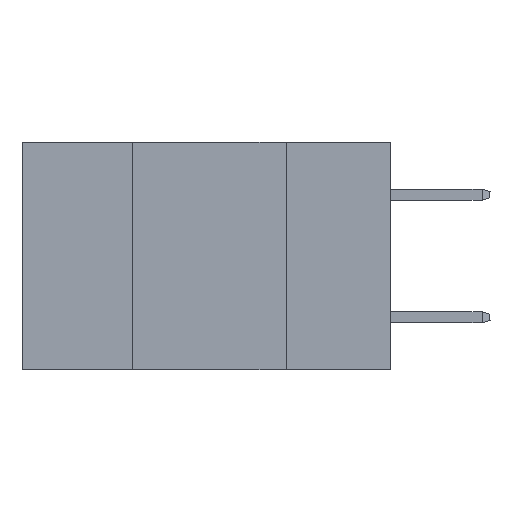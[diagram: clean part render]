
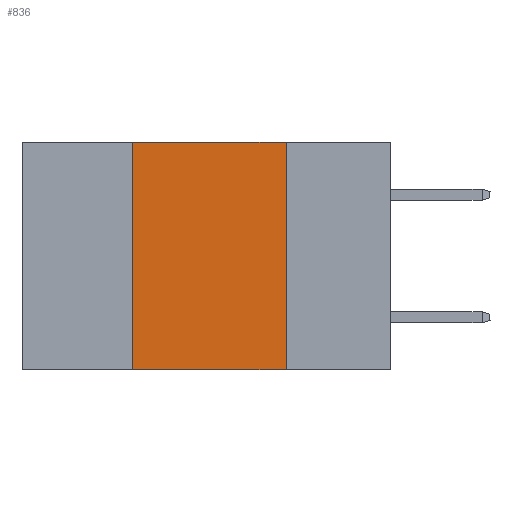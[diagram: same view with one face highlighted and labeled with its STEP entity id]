
A CAD part, left-side view. The second image highlights one B-rep face of the part: STEP entity #836.
In plain terms, the highlighted planar face has unit normal (-1, 0, 0).
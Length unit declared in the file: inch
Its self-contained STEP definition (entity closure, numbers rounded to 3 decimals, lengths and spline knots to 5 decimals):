
#183 = ORIENTED_EDGE ( 'NONE', *, *, #1083, .F. ) ;
#836 = ADVANCED_FACE ( 'NONE', ( #3090 ), #2883, .F. ) ;
#1083 = EDGE_CURVE ( 'NONE', #12648, #2559, #15707, .T. ) ;
#1104 = CARTESIAN_POINT ( 'NONE',  ( 0., 0.42, -0.37 ) ) ;
#1356 = DIRECTION ( 'NONE',  ( 0., -1., 0. ) ) ;
#1538 = EDGE_CURVE ( 'NONE', #8783, #17082, #5696, .T. ) ;
#1932 = VECTOR ( 'NONE', #1356, 39.37008 ) ;
#2559 = VERTEX_POINT ( 'NONE', #19711 ) ;
#2883 = PLANE ( 'NONE',  #14204 ) ;
#3090 = FACE_OUTER_BOUND ( 'NONE', #19800, .T. ) ;
#3466 = CARTESIAN_POINT ( 'NONE',  ( 0., 0.42, 0. ) ) ;
#3748 = EDGE_CURVE ( 'NONE', #12648, #17082, #10175, .T. ) ;
#4660 = CARTESIAN_POINT ( 'NONE',  ( 0., 0.17, -0.37 ) ) ;
#4738 = DIRECTION ( 'NONE',  ( 0., 0., -1. ) ) ;
#5691 = DIRECTION ( 'NONE',  ( 0., -1., 0. ) ) ;
#5696 = LINE ( 'NONE', #6058, #16393 ) ;
#5962 = VECTOR ( 'NONE', #6739, 39.37008 ) ;
#6058 = CARTESIAN_POINT ( 'NONE',  ( 0., 0.17, 0. ) ) ;
#6275 = VECTOR ( 'NONE', #5691, 39.37008 ) ;
#6739 = DIRECTION ( 'NONE',  ( 0., 0., 1. ) ) ;
#8783 = VERTEX_POINT ( 'NONE', #18754 ) ;
#9027 = ORIENTED_EDGE ( 'NONE', *, *, #11069, .F. ) ;
#10175 = LINE ( 'NONE', #11825, #6275 ) ;
#11069 = EDGE_CURVE ( 'NONE', #2559, #8783, #11654, .T. ) ;
#11654 = LINE ( 'NONE', #13685, #1932 ) ;
#11777 = ORIENTED_EDGE ( 'NONE', *, *, #1538, .F. ) ;
#11825 = CARTESIAN_POINT ( 'NONE',  ( 0., 0.6, -0.37 ) ) ;
#12648 = VERTEX_POINT ( 'NONE', #1104 ) ;
#13363 = ORIENTED_EDGE ( 'NONE', *, *, #3748, .T. ) ;
#13505 = CARTESIAN_POINT ( 'NONE',  ( 0., 0.6, 0. ) ) ;
#13685 = CARTESIAN_POINT ( 'NONE',  ( 0., 0.6, 0. ) ) ;
#14204 = AXIS2_PLACEMENT_3D ( 'NONE', #13505, #15864, #4738 ) ;
#15707 = LINE ( 'NONE', #3466, #5962 ) ;
#15864 = DIRECTION ( 'NONE',  ( 1., 0., 0. ) ) ;
#16393 = VECTOR ( 'NONE', #17022, 39.37008 ) ;
#17022 = DIRECTION ( 'NONE',  ( 0., 0., -1. ) ) ;
#17082 = VERTEX_POINT ( 'NONE', #4660 ) ;
#18754 = CARTESIAN_POINT ( 'NONE',  ( 0., 0.17, 0. ) ) ;
#19711 = CARTESIAN_POINT ( 'NONE',  ( 0., 0.42, 0. ) ) ;
#19800 = EDGE_LOOP ( 'NONE', ( #11777, #9027, #183, #13363 ) ) ;
